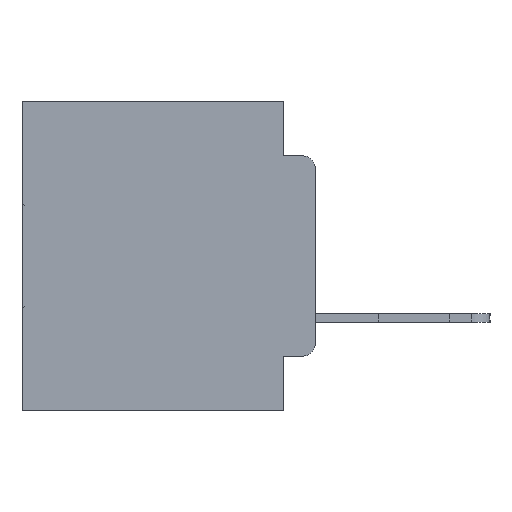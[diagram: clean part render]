
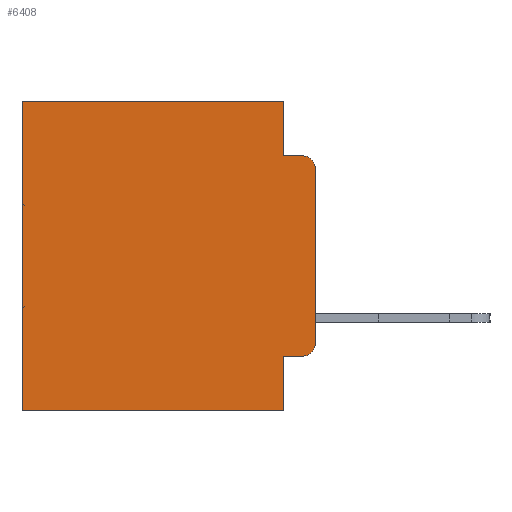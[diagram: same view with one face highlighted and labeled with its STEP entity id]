
A CAD part, left-side view. The second image highlights one B-rep face of the part: STEP entity #6408.
In plain terms, the highlighted planar face has unit normal (-1, 0, 0).
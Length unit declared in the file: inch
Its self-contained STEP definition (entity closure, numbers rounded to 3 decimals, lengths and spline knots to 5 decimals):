
#154 = ORIENTED_EDGE ( 'NONE', *, *, #15572, .F. ) ;
#462 = DIRECTION ( 'NONE',  ( 0., 0., -1. ) ) ;
#1123 = DIRECTION ( 'NONE',  ( 0., -1., 0. ) ) ;
#1272 = CARTESIAN_POINT ( 'NONE',  ( 0.298, 0.051, 0. ) ) ;
#1328 = VERTEX_POINT ( 'NONE', #6573 ) ;
#1790 = ORIENTED_EDGE ( 'NONE', *, *, #11748, .T. ) ;
#2748 = CARTESIAN_POINT ( 'NONE',  ( 0.298, 0.473, 0. ) ) ;
#3920 = ORIENTED_EDGE ( 'NONE', *, *, #18670, .T. ) ;
#4312 = LINE ( 'NONE', #18430, #29752 ) ;
#5797 = VERTEX_POINT ( 'NONE', #29555 ) ;
#6408 = ADVANCED_FACE ( 'NONE', ( #22645 ), #13998, .F. ) ;
#6481 = VECTOR ( 'NONE', #6724, 39.37008 ) ;
#6557 = VERTEX_POINT ( 'NONE', #29398 ) ;
#6573 = CARTESIAN_POINT ( 'NONE',  ( 0.298, 0., -0.1085 ) ) ;
#6724 = DIRECTION ( 'NONE',  ( 0., 0., -1. ) ) ;
#7586 = ORIENTED_EDGE ( 'NONE', *, *, #17780, .F. ) ;
#7799 = VERTEX_POINT ( 'NONE', #31046 ) ;
#9002 = DIRECTION ( 'NONE',  ( -1., 0., 0. ) ) ;
#9957 = ORIENTED_EDGE ( 'NONE', *, *, #26801, .T. ) ;
#10468 = ORIENTED_EDGE ( 'NONE', *, *, #22809, .F. ) ;
#10732 = CARTESIAN_POINT ( 'NONE',  ( 0.298, 0.02, -0.3915 ) ) ;
#11217 = AXIS2_PLACEMENT_3D ( 'NONE', #10732, #28143, #13394 ) ;
#11267 = CARTESIAN_POINT ( 'NONE',  ( 0.298, 0.051, 0. ) ) ;
#11323 = VERTEX_POINT ( 'NONE', #18124 ) ;
#11358 = DIRECTION ( 'NONE',  ( 0., 0., -1. ) ) ;
#11748 = EDGE_CURVE ( 'NONE', #14903, #5797, #26029, .T. ) ;
#11995 = CARTESIAN_POINT ( 'NONE',  ( 0.298, 0.051, -0.0885 ) ) ;
#12575 = ORIENTED_EDGE ( 'NONE', *, *, #27961, .T. ) ;
#12662 = VERTEX_POINT ( 'NONE', #20076 ) ;
#13255 = CIRCLE ( 'NONE', #20968, 0.02 ) ;
#13394 = DIRECTION ( 'NONE',  ( 0., 0., -1. ) ) ;
#13493 = VECTOR ( 'NONE', #27938, 39.37008 ) ;
#13998 = PLANE ( 'NONE',  #14392 ) ;
#14392 = AXIS2_PLACEMENT_3D ( 'NONE', #30949, #16580, #462 ) ;
#14903 = VERTEX_POINT ( 'NONE', #30706 ) ;
#14957 = VECTOR ( 'NONE', #11358, 39.37008 ) ;
#15354 = DIRECTION ( 'NONE',  ( 0., 0., -1. ) ) ;
#15572 = EDGE_CURVE ( 'NONE', #6557, #12662, #22436, .T. ) ;
#15948 = LINE ( 'NONE', #25632, #13493 ) ;
#16580 = DIRECTION ( 'NONE',  ( 1., 0., 0. ) ) ;
#17114 = CARTESIAN_POINT ( 'NONE',  ( 0.298, 0.02, -0.0885 ) ) ;
#17780 = EDGE_CURVE ( 'NONE', #30273, #7799, #26858, .T. ) ;
#18124 = CARTESIAN_POINT ( 'NONE',  ( 0.298, 0.051, -0.4115 ) ) ;
#18327 = CARTESIAN_POINT ( 'NONE',  ( 0.298, 0., -0.5 ) ) ;
#18430 = CARTESIAN_POINT ( 'NONE',  ( 0.298, 0., 0. ) ) ;
#18611 = EDGE_CURVE ( 'NONE', #11323, #6557, #27919, .T. ) ;
#18670 = EDGE_CURVE ( 'NONE', #1328, #22803, #13255, .T. ) ;
#19674 = CARTESIAN_POINT ( 'NONE',  ( 0.298, 0.051, -0.4115 ) ) ;
#20076 = CARTESIAN_POINT ( 'NONE',  ( 0.298, 0.473, -0.5 ) ) ;
#20297 = CARTESIAN_POINT ( 'NONE',  ( 0.298, 0., 0. ) ) ;
#20968 = AXIS2_PLACEMENT_3D ( 'NONE', #24209, #9002, #26634 ) ;
#22030 = ORIENTED_EDGE ( 'NONE', *, *, #24557, .T. ) ;
#22436 = LINE ( 'NONE', #18327, #28064 ) ;
#22645 = FACE_OUTER_BOUND ( 'NONE', #29353, .T. ) ;
#22803 = VERTEX_POINT ( 'NONE', #17114 ) ;
#22809 = EDGE_CURVE ( 'NONE', #7799, #22803, #32101, .T. ) ;
#24209 = CARTESIAN_POINT ( 'NONE',  ( 0.298, 0.02, -0.1085 ) ) ;
#24557 = EDGE_CURVE ( 'NONE', #30947, #12662, #15948, .T. ) ;
#24768 = VECTOR ( 'NONE', #15354, 39.37008 ) ;
#25005 = ORIENTED_EDGE ( 'NONE', *, *, #25200, .F. ) ;
#25200 = EDGE_CURVE ( 'NONE', #1328, #5797, #31014, .T. ) ;
#25632 = CARTESIAN_POINT ( 'NONE',  ( 0.298, 0.473, 0. ) ) ;
#25722 = LINE ( 'NONE', #19674, #26480 ) ;
#26029 = CIRCLE ( 'NONE', #11217, 0.02 ) ;
#26480 = VECTOR ( 'NONE', #1123, 39.37008 ) ;
#26634 = DIRECTION ( 'NONE',  ( 0., 0., -1. ) ) ;
#26801 = EDGE_CURVE ( 'NONE', #11323, #14903, #25722, .T. ) ;
#26858 = LINE ( 'NONE', #1272, #6481 ) ;
#27919 = LINE ( 'NONE', #28721, #14957 ) ;
#27938 = DIRECTION ( 'NONE',  ( 0., 0., -1. ) ) ;
#27961 = EDGE_CURVE ( 'NONE', #30273, #30947, #4312, .T. ) ;
#28064 = VECTOR ( 'NONE', #30395, 39.37008 ) ;
#28143 = DIRECTION ( 'NONE',  ( -1., 0., 0. ) ) ;
#28721 = CARTESIAN_POINT ( 'NONE',  ( 0.298, 0.051, 0. ) ) ;
#29273 = DIRECTION ( 'NONE',  ( 0., -1., 0. ) ) ;
#29353 = EDGE_LOOP ( 'NONE', ( #25005, #3920, #10468, #7586, #12575, #22030, #154, #31870, #9957, #1790 ) ) ;
#29398 = CARTESIAN_POINT ( 'NONE',  ( 0.298, 0.051, -0.5 ) ) ;
#29555 = CARTESIAN_POINT ( 'NONE',  ( 0.298, 0., -0.3915 ) ) ;
#29752 = VECTOR ( 'NONE', #32613, 39.37008 ) ;
#30273 = VERTEX_POINT ( 'NONE', #11267 ) ;
#30395 = DIRECTION ( 'NONE',  ( 0., 1., 0. ) ) ;
#30706 = CARTESIAN_POINT ( 'NONE',  ( 0.298, 0.02, -0.4115 ) ) ;
#30721 = VECTOR ( 'NONE', #29273, 39.37008 ) ;
#30947 = VERTEX_POINT ( 'NONE', #2748 ) ;
#30949 = CARTESIAN_POINT ( 'NONE',  ( 0.298, 0., 0. ) ) ;
#31014 = LINE ( 'NONE', #20297, #24768 ) ;
#31046 = CARTESIAN_POINT ( 'NONE',  ( 0.298, 0.051, -0.0885 ) ) ;
#31870 = ORIENTED_EDGE ( 'NONE', *, *, #18611, .F. ) ;
#32101 = LINE ( 'NONE', #11995, #30721 ) ;
#32613 = DIRECTION ( 'NONE',  ( 0., 1., 0. ) ) ;
